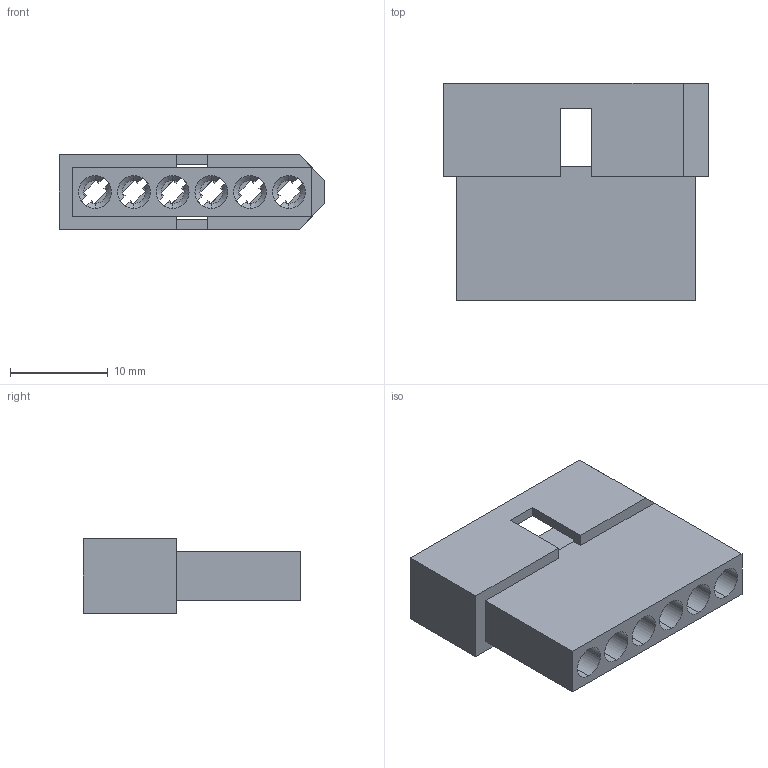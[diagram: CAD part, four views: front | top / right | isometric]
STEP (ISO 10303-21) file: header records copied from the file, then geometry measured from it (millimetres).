
FILE_DESCRIPTION (( 'STEP AP203' ), '1' );
FILE_NAME ('556-006-000-201.STEP', '2020-03-13T15:08:55', ( '' ), ( '' ), 'SwSTEP 2.0', 'SolidWorks 2016', '' );
FILE_SCHEMA (( 'CONFIG_CONTROL_DESIGN' ));
Length unit declared in the file: millimetre
Products named in the file (2): 556-210-001_556-006-000-201; 556-006-000-201
Assembly tree (1 placements, depth 2):
  556-006-000-201
    556-210-001_556-006-000-201
Bounding box: 27.13 x 22.23 x 7.62 mm (x, y, z)
Volume: 1676.1 mm3; surface area: 3070.2 mm2
Topology: 1 solids, 1 shells, 185 faces, 542 edges, 356 vertices
Faces by surface type: plane 137, cylinder 36, cone 12
Entity records: 6408 total; most frequent: CARTESIAN_POINT 1303, ORIENTED_EDGE 1084, DIRECTION 968, EDGE_CURVE 542, VERTEX_POINT 356, LINE 350, VECTOR 350, AXIS2_PLACEMENT_3D 309
